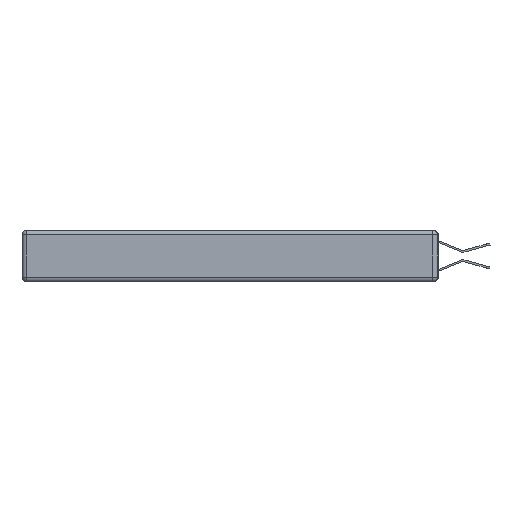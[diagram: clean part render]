
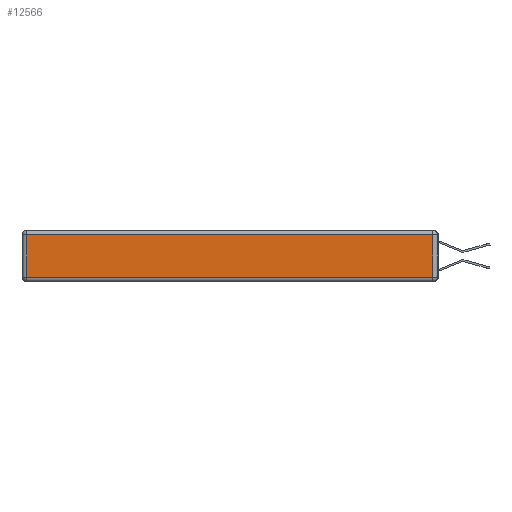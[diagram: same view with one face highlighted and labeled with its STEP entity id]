
A CAD part, left-side view. The second image highlights one B-rep face of the part: STEP entity #12566.
In plain terms, the highlighted planar face has unit normal (-1, 0, 0).
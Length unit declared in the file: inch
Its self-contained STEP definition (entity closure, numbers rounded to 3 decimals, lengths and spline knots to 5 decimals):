
#384 = EDGE_CURVE ( 'NONE', #18150, #2013, #8742, .T. ) ;
#1110 = FACE_OUTER_BOUND ( 'NONE', #12864, .T. ) ;
#1605 = ORIENTED_EDGE ( 'NONE', *, *, #7824, .T. ) ;
#2013 = VERTEX_POINT ( 'NONE', #3443 ) ;
#3443 = CARTESIAN_POINT ( 'NONE',  ( 0., 0.03, -0.03 ) ) ;
#3566 = VERTEX_POINT ( 'NONE', #17536 ) ;
#4200 = VERTEX_POINT ( 'NONE', #13825 ) ;
#5883 = VECTOR ( 'NONE', #18754, 39.37008 ) ;
#6005 = LINE ( 'NONE', #20465, #5883 ) ;
#7824 = EDGE_CURVE ( 'NONE', #4200, #3566, #7996, .T. ) ;
#7996 = LINE ( 'NONE', #17432, #18906 ) ;
#8093 = VECTOR ( 'NONE', #16231, 39.37008 ) ;
#8499 = DIRECTION ( 'NONE',  ( -1., 0., 0. ) ) ;
#8742 = LINE ( 'NONE', #12795, #8093 ) ;
#9510 = DIRECTION ( 'NONE',  ( 0., 0., -1. ) ) ;
#10990 = ORIENTED_EDGE ( 'NONE', *, *, #384, .T. ) ;
#12316 = CARTESIAN_POINT ( 'NONE',  ( 0., 0., -0.343 ) ) ;
#12368 = ORIENTED_EDGE ( 'NONE', *, *, #19164, .T. ) ;
#12566 = ADVANCED_FACE ( 'NONE', ( #1110 ), #14171, .T. ) ;
#12795 = CARTESIAN_POINT ( 'NONE',  ( 0., 0.03, -0.343 ) ) ;
#12864 = EDGE_LOOP ( 'NONE', ( #12368, #10990, #23931, #1605 ) ) ;
#13825 = CARTESIAN_POINT ( 'NONE',  ( 0., 2.72, -0.03 ) ) ;
#14171 = PLANE ( 'NONE',  #14179 ) ;
#14179 = AXIS2_PLACEMENT_3D ( 'NONE', #12316, #8499, #15993 ) ;
#15993 = DIRECTION ( 'NONE',  ( 0., 0., 1. ) ) ;
#16231 = DIRECTION ( 'NONE',  ( 0., 0., 1. ) ) ;
#17432 = CARTESIAN_POINT ( 'NONE',  ( 0., 2.72, -0.343 ) ) ;
#17536 = CARTESIAN_POINT ( 'NONE',  ( 0., 2.72, -0.313 ) ) ;
#18150 = VERTEX_POINT ( 'NONE', #21210 ) ;
#18754 = DIRECTION ( 'NONE',  ( 0., 1., 0. ) ) ;
#18761 = CARTESIAN_POINT ( 'NONE',  ( 0., 0., -0.313 ) ) ;
#18906 = VECTOR ( 'NONE', #9510, 39.37008 ) ;
#19164 = EDGE_CURVE ( 'NONE', #3566, #18150, #24040, .T. ) ;
#20465 = CARTESIAN_POINT ( 'NONE',  ( 0., 2.75, -0.03 ) ) ;
#20596 = VECTOR ( 'NONE', #21951, 39.37008 ) ;
#21210 = CARTESIAN_POINT ( 'NONE',  ( 0., 0.03, -0.313 ) ) ;
#21951 = DIRECTION ( 'NONE',  ( 0., -1., 0. ) ) ;
#23931 = ORIENTED_EDGE ( 'NONE', *, *, #24012, .T. ) ;
#24012 = EDGE_CURVE ( 'NONE', #2013, #4200, #6005, .T. ) ;
#24040 = LINE ( 'NONE', #18761, #20596 ) ;
